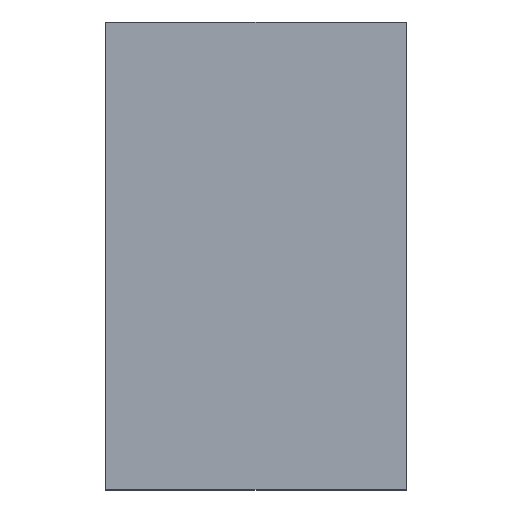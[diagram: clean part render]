
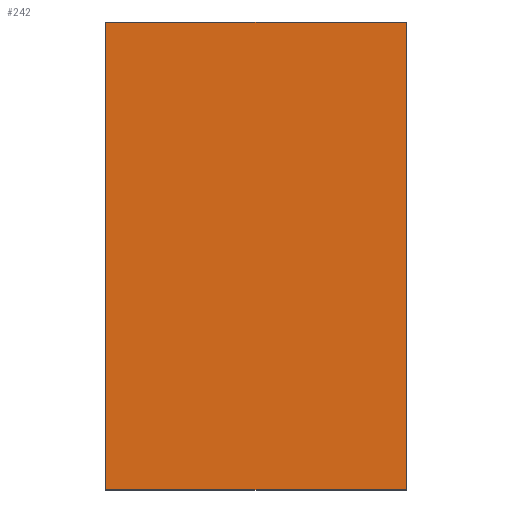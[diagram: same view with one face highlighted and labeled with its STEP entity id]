
A CAD part, top view. The second image highlights one B-rep face of the part: STEP entity #242.
In plain terms, the highlighted planar face has unit normal (0, 0, 1).
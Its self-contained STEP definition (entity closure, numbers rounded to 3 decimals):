
#14 = CARTESIAN_POINT ( 'NONE',  ( -13.436, -41.834, 14.305 ) ) ;
#43 = FACE_OUTER_BOUND ( 'NONE', #835, .T. ) ;
#142 = CARTESIAN_POINT ( 'NONE',  ( 13.439, 0., 14.305 ) ) ;
#176 = VECTOR ( 'NONE', #735, 1000. ) ;
#179 = VERTEX_POINT ( 'NONE', #480 ) ;
#201 = ORIENTED_EDGE ( 'NONE', *, *, #386, .T. ) ;
#217 = DIRECTION ( 'NONE',  ( 0., -1., 0. ) ) ;
#230 = EDGE_CURVE ( 'NONE', #179, #709, #625, .T. ) ;
#242 = ADVANCED_FACE ( 'NONE', ( #43 ), #630, .T. ) ;
#263 = DIRECTION ( 'NONE',  ( 0., 0., 1. ) ) ;
#279 = CARTESIAN_POINT ( 'NONE',  ( -13.436, 0., 14.305 ) ) ;
#307 = EDGE_CURVE ( 'NONE', #709, #468, #595, .T. ) ;
#344 = DIRECTION ( 'NONE',  ( 0., 1., 0. ) ) ;
#358 = DIRECTION ( 'NONE',  ( 1., 0., 0. ) ) ;
#386 = EDGE_CURVE ( 'NONE', #468, #479, #939, .T. ) ;
#402 = ORIENTED_EDGE ( 'NONE', *, *, #307, .T. ) ;
#413 = ORIENTED_EDGE ( 'NONE', *, *, #230, .T. ) ;
#415 = AXIS2_PLACEMENT_3D ( 'NONE', #490, #263, #469 ) ;
#437 = LINE ( 'NONE', #952, #499 ) ;
#468 = VERTEX_POINT ( 'NONE', #538 ) ;
#469 = DIRECTION ( 'NONE',  ( 1., 0., 0. ) ) ;
#474 = CARTESIAN_POINT ( 'NONE',  ( 13.439, -41.834, 14.305 ) ) ;
#479 = VERTEX_POINT ( 'NONE', #14 ) ;
#480 = CARTESIAN_POINT ( 'NONE',  ( 13.439, -41.834, 14.305 ) ) ;
#490 = CARTESIAN_POINT ( 'NONE',  ( 0., 0., 14.305 ) ) ;
#499 = VECTOR ( 'NONE', #358, 1000. ) ;
#514 = CARTESIAN_POINT ( 'NONE',  ( 13.439, 0., 14.305 ) ) ;
#538 = CARTESIAN_POINT ( 'NONE',  ( -13.436, 0., 14.305 ) ) ;
#569 = ORIENTED_EDGE ( 'NONE', *, *, #642, .T. ) ;
#595 = LINE ( 'NONE', #514, #176 ) ;
#625 = LINE ( 'NONE', #474, #885 ) ;
#630 = PLANE ( 'NONE',  #415 ) ;
#642 = EDGE_CURVE ( 'NONE', #479, #179, #437, .T. ) ;
#709 = VERTEX_POINT ( 'NONE', #142 ) ;
#735 = DIRECTION ( 'NONE',  ( -1., 0., 0. ) ) ;
#835 = EDGE_LOOP ( 'NONE', ( #569, #413, #402, #201 ) ) ;
#885 = VECTOR ( 'NONE', #344, 1000. ) ;
#934 = VECTOR ( 'NONE', #217, 1000. ) ;
#939 = LINE ( 'NONE', #279, #934 ) ;
#952 = CARTESIAN_POINT ( 'NONE',  ( -13.436, -41.834, 14.305 ) ) ;
